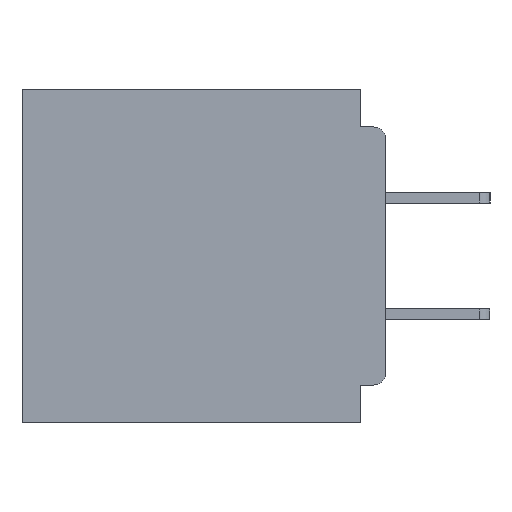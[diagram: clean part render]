
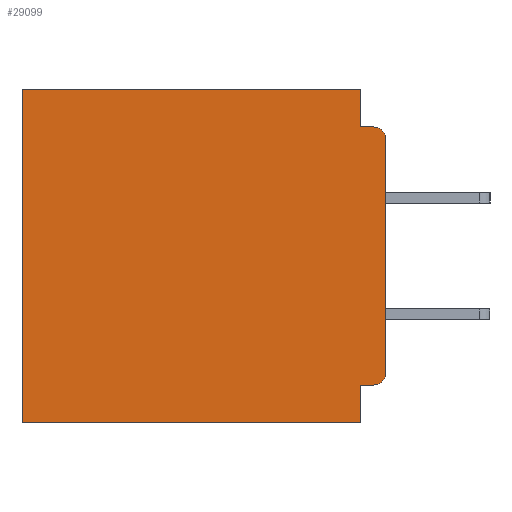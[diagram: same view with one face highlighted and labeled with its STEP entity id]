
A CAD part, left-side view. The second image highlights one B-rep face of the part: STEP entity #29099.
In plain terms, the highlighted planar face has unit normal (-1, 0, 0).
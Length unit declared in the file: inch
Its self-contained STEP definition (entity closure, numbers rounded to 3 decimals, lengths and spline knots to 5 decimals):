
#464 = LINE ( 'NONE', #13549, #42573 ) ;
#797 = VERTEX_POINT ( 'NONE', #32542 ) ;
#3085 = DIRECTION ( 'NONE',  ( -1., 0., 0. ) ) ;
#3535 = DIRECTION ( 'NONE',  ( 0., 0., -1. ) ) ;
#4966 = VERTEX_POINT ( 'NONE', #22237 ) ;
#5259 = LINE ( 'NONE', #9800, #25709 ) ;
#5382 = VECTOR ( 'NONE', #27003, 39.37008 ) ;
#5733 = EDGE_CURVE ( 'NONE', #797, #27417, #5259, .T. ) ;
#5935 = CARTESIAN_POINT ( 'NONE',  ( 0.3, 0.015, -0.06 ) ) ;
#6198 = VECTOR ( 'NONE', #26495, 39.37008 ) ;
#6505 = CARTESIAN_POINT ( 'NONE',  ( 0.3, 0., -0.355 ) ) ;
#6984 = VERTEX_POINT ( 'NONE', #39922 ) ;
#8030 = EDGE_CURVE ( 'NONE', #33203, #22861, #39436, .T. ) ;
#8726 = ORIENTED_EDGE ( 'NONE', *, *, #20824, .F. ) ;
#9800 = CARTESIAN_POINT ( 'NONE',  ( 0.3, 0.437, -0.4 ) ) ;
#9976 = CARTESIAN_POINT ( 'NONE',  ( 0.3, 0.437, -0.4 ) ) ;
#10018 = DIRECTION ( 'NONE',  ( 0., 0., -1. ) ) ;
#10403 = DIRECTION ( 'NONE',  ( 0., 1., 0. ) ) ;
#10481 = ORIENTED_EDGE ( 'NONE', *, *, #16484, .F. ) ;
#10575 = VECTOR ( 'NONE', #34304, 39.37008 ) ;
#11178 = LINE ( 'NONE', #6505, #20820 ) ;
#11507 = CARTESIAN_POINT ( 'NONE',  ( 0.3, 0., -0.4 ) ) ;
#12870 = AXIS2_PLACEMENT_3D ( 'NONE', #33270, #37490, #13022 ) ;
#13022 = DIRECTION ( 'NONE',  ( 0., 0., -1. ) ) ;
#13549 = CARTESIAN_POINT ( 'NONE',  ( 0.3, 0., 0. ) ) ;
#14006 = ORIENTED_EDGE ( 'NONE', *, *, #26835, .F. ) ;
#14874 = VECTOR ( 'NONE', #16512, 39.37008 ) ;
#14912 = EDGE_CURVE ( 'NONE', #6984, #28287, #38766, .T. ) ;
#15227 = CARTESIAN_POINT ( 'NONE',  ( 0.3, 0.015, -0.045 ) ) ;
#16484 = EDGE_CURVE ( 'NONE', #4966, #44574, #27047, .T. ) ;
#16512 = DIRECTION ( 'NONE',  ( 0., 0., -1. ) ) ;
#20820 = VECTOR ( 'NONE', #10403, 39.37008 ) ;
#20824 = EDGE_CURVE ( 'NONE', #28763, #6984, #11178, .T. ) ;
#21485 = LINE ( 'NONE', #46436, #10575 ) ;
#22237 = CARTESIAN_POINT ( 'NONE',  ( 0.3, 0.031, 0. ) ) ;
#22376 = CARTESIAN_POINT ( 'NONE',  ( 0.3, 0.031, -0.4 ) ) ;
#22861 = VERTEX_POINT ( 'NONE', #15227 ) ;
#23051 = AXIS2_PLACEMENT_3D ( 'NONE', #27536, #3085, #31648 ) ;
#23082 = CARTESIAN_POINT ( 'NONE',  ( 0.3, 0.015, -0.355 ) ) ;
#25233 = PLANE ( 'NONE',  #12870 ) ;
#25709 = VECTOR ( 'NONE', #25868, 39.37008 ) ;
#25868 = DIRECTION ( 'NONE',  ( 0., 0., -1. ) ) ;
#26495 = DIRECTION ( 'NONE',  ( 0., 0., -1. ) ) ;
#26835 = EDGE_CURVE ( 'NONE', #28287, #27417, #36648, .T. ) ;
#26937 = EDGE_CURVE ( 'NONE', #28763, #42640, #43582, .T. ) ;
#27003 = DIRECTION ( 'NONE',  ( 0., 1., 0. ) ) ;
#27047 = LINE ( 'NONE', #44976, #14874 ) ;
#27417 = VERTEX_POINT ( 'NONE', #9976 ) ;
#27536 = CARTESIAN_POINT ( 'NONE',  ( 0.3, 0.015, -0.34 ) ) ;
#28287 = VERTEX_POINT ( 'NONE', #48677 ) ;
#28763 = VERTEX_POINT ( 'NONE', #23082 ) ;
#29099 = ADVANCED_FACE ( 'NONE', ( #43626 ), #25233, .F. ) ;
#31322 = EDGE_LOOP ( 'NONE', ( #38123, #50300, #47352, #10481, #33111, #40648, #14006, #39137, #8726, #42737 ) ) ;
#31648 = DIRECTION ( 'NONE',  ( 0., 0., -1. ) ) ;
#32523 = VECTOR ( 'NONE', #3535, 39.37008 ) ;
#32542 = CARTESIAN_POINT ( 'NONE',  ( 0.3, 0.437, 0. ) ) ;
#33111 = ORIENTED_EDGE ( 'NONE', *, *, #43856, .T. ) ;
#33203 = VERTEX_POINT ( 'NONE', #34075 ) ;
#33270 = CARTESIAN_POINT ( 'NONE',  ( 0.3, 0., -0.4 ) ) ;
#33986 = DIRECTION ( 'NONE',  ( 0., 1., 0. ) ) ;
#34075 = CARTESIAN_POINT ( 'NONE',  ( 0.3, 0., -0.06 ) ) ;
#34304 = DIRECTION ( 'NONE',  ( 0., -1., 0. ) ) ;
#34526 = DIRECTION ( 'NONE',  ( -1., 0., 0. ) ) ;
#36648 = LINE ( 'NONE', #51255, #5382 ) ;
#36740 = EDGE_CURVE ( 'NONE', #33203, #42640, #43274, .T. ) ;
#37490 = DIRECTION ( 'NONE',  ( 1., 0., 0. ) ) ;
#38123 = ORIENTED_EDGE ( 'NONE', *, *, #36740, .F. ) ;
#38766 = LINE ( 'NONE', #22376, #6198 ) ;
#39137 = ORIENTED_EDGE ( 'NONE', *, *, #14912, .F. ) ;
#39436 = CIRCLE ( 'NONE', #40117, 0.015 ) ;
#39922 = CARTESIAN_POINT ( 'NONE',  ( 0.3, 0.031, -0.355 ) ) ;
#40117 = AXIS2_PLACEMENT_3D ( 'NONE', #5935, #34526, #10018 ) ;
#40648 = ORIENTED_EDGE ( 'NONE', *, *, #5733, .T. ) ;
#42573 = VECTOR ( 'NONE', #33986, 39.37008 ) ;
#42578 = CARTESIAN_POINT ( 'NONE',  ( 0.3, 0., -0.34 ) ) ;
#42640 = VERTEX_POINT ( 'NONE', #42578 ) ;
#42737 = ORIENTED_EDGE ( 'NONE', *, *, #26937, .T. ) ;
#43274 = LINE ( 'NONE', #11507, #32523 ) ;
#43582 = CIRCLE ( 'NONE', #23051, 0.015 ) ;
#43626 = FACE_OUTER_BOUND ( 'NONE', #31322, .T. ) ;
#43856 = EDGE_CURVE ( 'NONE', #4966, #797, #464, .T. ) ;
#44471 = EDGE_CURVE ( 'NONE', #44574, #22861, #21485, .T. ) ;
#44574 = VERTEX_POINT ( 'NONE', #51175 ) ;
#44976 = CARTESIAN_POINT ( 'NONE',  ( 0.3, 0.031, 0. ) ) ;
#46436 = CARTESIAN_POINT ( 'NONE',  ( 0.3, 0., -0.045 ) ) ;
#47352 = ORIENTED_EDGE ( 'NONE', *, *, #44471, .F. ) ;
#48677 = CARTESIAN_POINT ( 'NONE',  ( 0.3, 0.031, -0.4 ) ) ;
#50300 = ORIENTED_EDGE ( 'NONE', *, *, #8030, .T. ) ;
#51175 = CARTESIAN_POINT ( 'NONE',  ( 0.3, 0.031, -0.045 ) ) ;
#51255 = CARTESIAN_POINT ( 'NONE',  ( 0.3, 0., -0.4 ) ) ;
